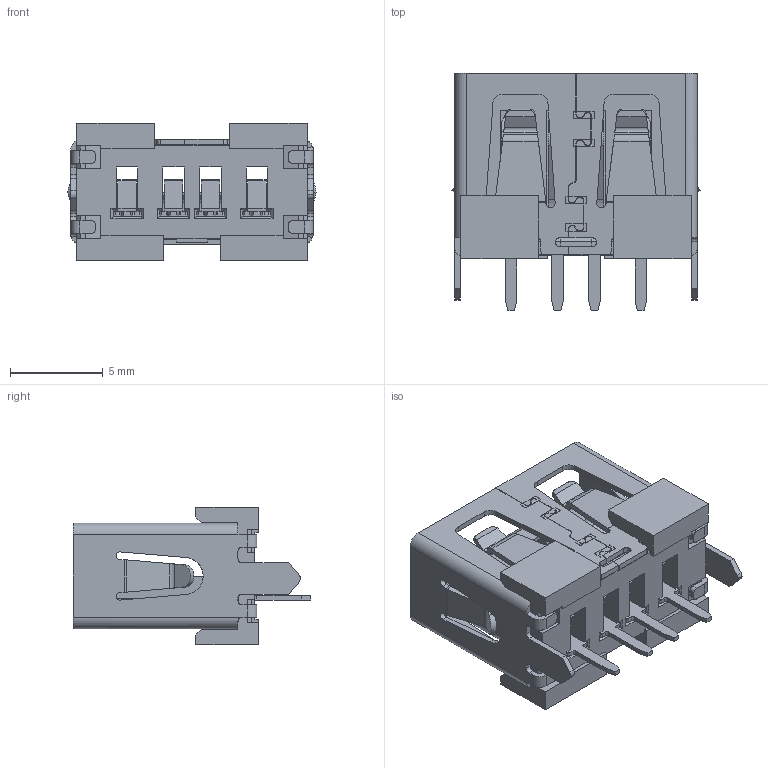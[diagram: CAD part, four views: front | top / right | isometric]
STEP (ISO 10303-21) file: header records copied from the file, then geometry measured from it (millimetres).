
FILE_DESCRIPTION (( 'STEP AP214' ), '1' );
FILE_NAME ('690E104-141-611.STEP', '2021-01-14T12:34:07', ( '' ), ( '' ), 'SwSTEP 2.0', 'SolidWorks 2020', '' );
FILE_SCHEMA (( 'AUTOMOTIVE_DESIGN' ));
Length unit declared in the file: millimetre
Products named in the file (4): Contacts 690E104-141-611; 690E104-141-611; Shell 690E104-141-611; Insulator 690E104-141-611
Assembly tree (3 placements, depth 2):
  690E104-141-611
    Insulator 690E104-141-611
    Contacts 690E104-141-611
    Shell 690E104-141-611
Bounding box: 13.39 x 12.8 x 7.4 mm (x, y, z)
Volume: 321 mm3; surface area: 1418.9 mm2
Topology: 6 solids, 6 shells, 793 faces, 2270 edges, 1486 vertices
Faces by surface type: plane 552, cylinder 217, bspline 20, cone 4
Entity records: 26675 total; most frequent: CARTESIAN_POINT 5776, ORIENTED_EDGE 4540, DIRECTION 4042, EDGE_CURVE 2270, LINE 1780, VECTOR 1780, VERTEX_POINT 1486, AXIS2_PLACEMENT_3D 1131
